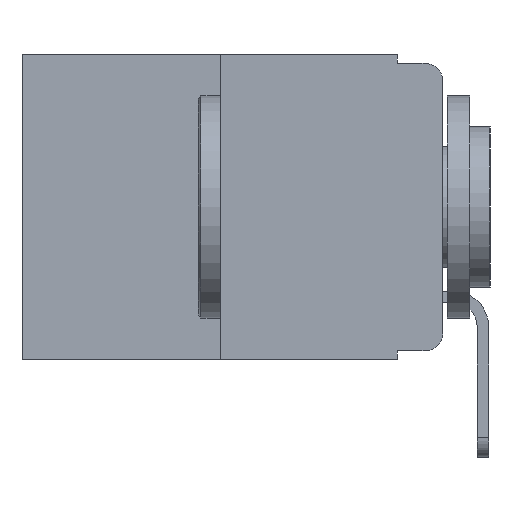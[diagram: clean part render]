
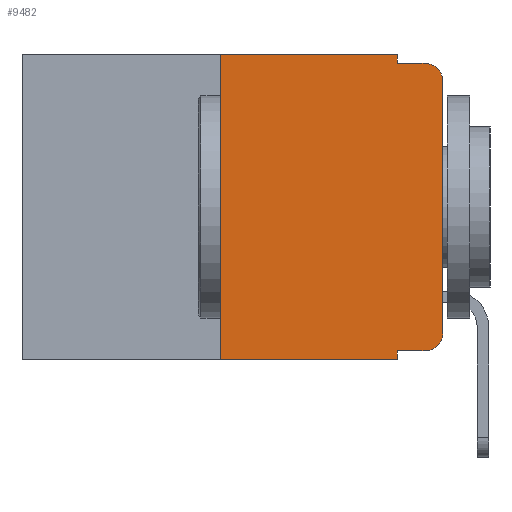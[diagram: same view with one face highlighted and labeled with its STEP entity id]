
A CAD part, left-side view. The second image highlights one B-rep face of the part: STEP entity #9482.
In plain terms, the highlighted planar face has unit normal (-1, 0, 0).
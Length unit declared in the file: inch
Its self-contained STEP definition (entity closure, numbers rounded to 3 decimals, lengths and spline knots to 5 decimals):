
#4 = VECTOR ( 'NONE', #13254, 39.37008 ) ;
#76 = VECTOR ( 'NONE', #3436, 39.37008 ) ;
#99 = LINE ( 'NONE', #14424, #1294 ) ;
#200 = LINE ( 'NONE', #5805, #4 ) ;
#311 = CARTESIAN_POINT ( 'NONE',  ( 0., 0.02, -0.03 ) ) ;
#376 = DIRECTION ( 'NONE',  ( 0., 0., -1. ) ) ;
#517 = DIRECTION ( 'NONE',  ( -1., 0., 0. ) ) ;
#693 = VECTOR ( 'NONE', #4570, 39.37008 ) ;
#862 = VECTOR ( 'NONE', #10420, 39.37008 ) ;
#937 = CARTESIAN_POINT ( 'NONE',  ( 0., 0.25, 0. ) ) ;
#945 = VERTEX_POINT ( 'NONE', #12079 ) ;
#1059 = ORIENTED_EDGE ( 'NONE', *, *, #14183, .T. ) ;
#1093 = CARTESIAN_POINT ( 'NONE',  ( 0., 0.051, 0. ) ) ;
#1149 = ORIENTED_EDGE ( 'NONE', *, *, #13395, .T. ) ;
#1294 = VECTOR ( 'NONE', #3618, 39.37008 ) ;
#1480 = AXIS2_PLACEMENT_3D ( 'NONE', #6873, #13463, #5646 ) ;
#1568 = CARTESIAN_POINT ( 'NONE',  ( 0., 0.25, 0. ) ) ;
#1589 = CARTESIAN_POINT ( 'NONE',  ( 0., 0., -0.03 ) ) ;
#3130 = VECTOR ( 'NONE', #5707, 39.37008 ) ;
#3436 = DIRECTION ( 'NONE',  ( 0., 0., 1. ) ) ;
#3618 = DIRECTION ( 'NONE',  ( 0., -1., 0. ) ) ;
#4040 = ORIENTED_EDGE ( 'NONE', *, *, #10066, .T. ) ;
#4290 = VERTEX_POINT ( 'NONE', #13183 ) ;
#4371 = EDGE_CURVE ( 'NONE', #7716, #4290, #200, .T. ) ;
#4445 = EDGE_CURVE ( 'NONE', #945, #7537, #5590, .T. ) ;
#4570 = DIRECTION ( 'NONE',  ( 0., 0., -1. ) ) ;
#5037 = CIRCLE ( 'NONE', #11783, 0.02 ) ;
#5219 = ORIENTED_EDGE ( 'NONE', *, *, #4371, .F. ) ;
#5590 = LINE ( 'NONE', #1093, #693 ) ;
#5646 = DIRECTION ( 'NONE',  ( 0., 0., -1. ) ) ;
#5707 = DIRECTION ( 'NONE',  ( 0., -1., 0. ) ) ;
#5805 = CARTESIAN_POINT ( 'NONE',  ( 0., 0.051, 0. ) ) ;
#6620 = DIRECTION ( 'NONE',  ( 0., -1., 0. ) ) ;
#6796 = VECTOR ( 'NONE', #6620, 39.37008 ) ;
#6873 = CARTESIAN_POINT ( 'NONE',  ( 0., 0.473, 0. ) ) ;
#6934 = CARTESIAN_POINT ( 'NONE',  ( 0., 0.051, -0.333 ) ) ;
#7081 = DIRECTION ( 'NONE',  ( 0., 0., 1. ) ) ;
#7090 = AXIS2_PLACEMENT_3D ( 'NONE', #13965, #10576, #11441 ) ;
#7207 = VERTEX_POINT ( 'NONE', #10197 ) ;
#7537 = VERTEX_POINT ( 'NONE', #12436 ) ;
#7716 = VERTEX_POINT ( 'NONE', #8045 ) ;
#8045 = CARTESIAN_POINT ( 'NONE',  ( 0., 0.051, -0.333 ) ) ;
#8383 = CARTESIAN_POINT ( 'NONE',  ( 0., 0., -0.313 ) ) ;
#8472 = ORIENTED_EDGE ( 'NONE', *, *, #9955, .T. ) ;
#8703 = VECTOR ( 'NONE', #7081, 39.37008 ) ;
#8907 = LINE ( 'NONE', #6934, #3130 ) ;
#8991 = PLANE ( 'NONE',  #1480 ) ;
#9090 = CARTESIAN_POINT ( 'NONE',  ( 0., 0., 0. ) ) ;
#9099 = ORIENTED_EDGE ( 'NONE', *, *, #9835, .T. ) ;
#9162 = LINE ( 'NONE', #9090, #76 ) ;
#9180 = VERTEX_POINT ( 'NONE', #11425 ) ;
#9210 = ORIENTED_EDGE ( 'NONE', *, *, #10425, .F. ) ;
#9482 = ADVANCED_FACE ( 'NONE', ( #9713 ), #8991, .F. ) ;
#9676 = EDGE_CURVE ( 'NONE', #7207, #11252, #12795, .T. ) ;
#9713 = FACE_OUTER_BOUND ( 'NONE', #13305, .T. ) ;
#9835 = EDGE_CURVE ( 'NONE', #7207, #4290, #99, .T. ) ;
#9955 = EDGE_CURVE ( 'NONE', #12751, #14406, #11518, .T. ) ;
#10066 = EDGE_CURVE ( 'NONE', #10949, #9180, #5037, .T. ) ;
#10197 = CARTESIAN_POINT ( 'NONE',  ( 0., 0.25, -0.343 ) ) ;
#10420 = DIRECTION ( 'NONE',  ( 0., -1., 0. ) ) ;
#10425 = EDGE_CURVE ( 'NONE', #11252, #945, #13952, .T. ) ;
#10495 = CARTESIAN_POINT ( 'NONE',  ( 0., 0.473, 0. ) ) ;
#10576 = DIRECTION ( 'NONE',  ( -1., 0., 0. ) ) ;
#10949 = VERTEX_POINT ( 'NONE', #1589 ) ;
#11024 = ORIENTED_EDGE ( 'NONE', *, *, #9676, .F. ) ;
#11252 = VERTEX_POINT ( 'NONE', #937 ) ;
#11425 = CARTESIAN_POINT ( 'NONE',  ( 0., 0.02, -0.01 ) ) ;
#11441 = DIRECTION ( 'NONE',  ( 0., 0., -1. ) ) ;
#11518 = CIRCLE ( 'NONE', #7090, 0.02 ) ;
#11783 = AXIS2_PLACEMENT_3D ( 'NONE', #311, #517, #376 ) ;
#12079 = CARTESIAN_POINT ( 'NONE',  ( 0., 0.051, 0. ) ) ;
#12436 = CARTESIAN_POINT ( 'NONE',  ( 0., 0.051, -0.01 ) ) ;
#12751 = VERTEX_POINT ( 'NONE', #13003 ) ;
#12795 = LINE ( 'NONE', #1568, #8703 ) ;
#12950 = ORIENTED_EDGE ( 'NONE', *, *, #4445, .F. ) ;
#13003 = CARTESIAN_POINT ( 'NONE',  ( 0., 0.02, -0.333 ) ) ;
#13183 = CARTESIAN_POINT ( 'NONE',  ( 0., 0.051, -0.343 ) ) ;
#13199 = CARTESIAN_POINT ( 'NONE',  ( 0., 0.051, -0.01 ) ) ;
#13254 = DIRECTION ( 'NONE',  ( 0., 0., -1. ) ) ;
#13290 = EDGE_CURVE ( 'NONE', #7537, #9180, #14397, .T. ) ;
#13305 = EDGE_LOOP ( 'NONE', ( #1149, #4040, #13747, #12950, #9210, #11024, #9099, #5219, #1059, #8472 ) ) ;
#13395 = EDGE_CURVE ( 'NONE', #14406, #10949, #9162, .T. ) ;
#13463 = DIRECTION ( 'NONE',  ( 1., 0., 0. ) ) ;
#13747 = ORIENTED_EDGE ( 'NONE', *, *, #13290, .F. ) ;
#13952 = LINE ( 'NONE', #10495, #862 ) ;
#13965 = CARTESIAN_POINT ( 'NONE',  ( 0., 0.02, -0.313 ) ) ;
#14183 = EDGE_CURVE ( 'NONE', #7716, #12751, #8907, .T. ) ;
#14397 = LINE ( 'NONE', #13199, #6796 ) ;
#14406 = VERTEX_POINT ( 'NONE', #8383 ) ;
#14424 = CARTESIAN_POINT ( 'NONE',  ( 0., 0.473, -0.343 ) ) ;
